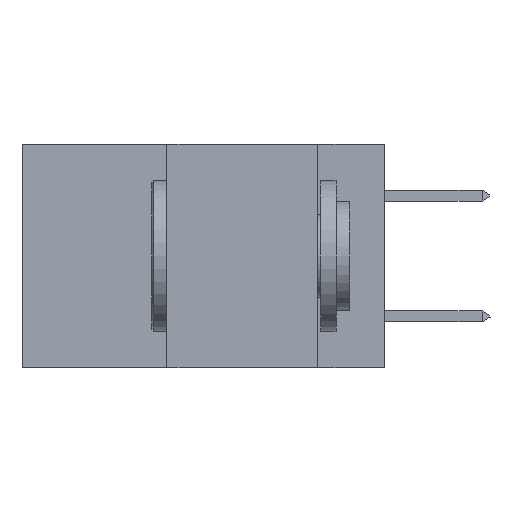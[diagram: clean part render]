
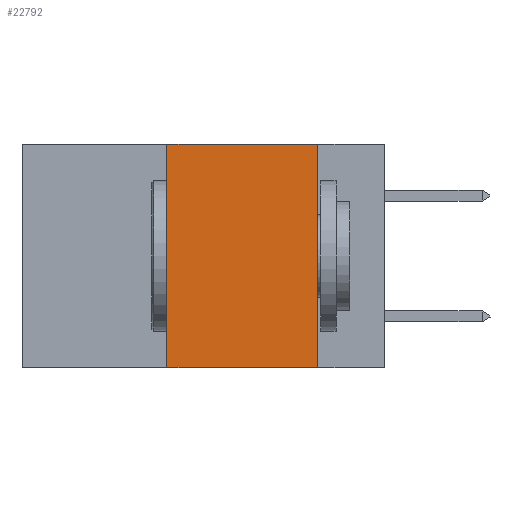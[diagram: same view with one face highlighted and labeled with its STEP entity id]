
A CAD part, left-side view. The second image highlights one B-rep face of the part: STEP entity #22792.
In plain terms, the highlighted planar face has unit normal (-1, 0, 0).
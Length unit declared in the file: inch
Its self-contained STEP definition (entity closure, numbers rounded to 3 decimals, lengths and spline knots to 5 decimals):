
#1737 = AXIS2_PLACEMENT_3D ( 'NONE', #43997, #23491, #2506 ) ;
#1740 = LINE ( 'NONE', #30843, #27474 ) ;
#2506 = DIRECTION ( 'NONE',  ( 0., 0., -1. ) ) ;
#3449 = ORIENTED_EDGE ( 'NONE', *, *, #29821, .T. ) ;
#3748 = VERTEX_POINT ( 'NONE', #8280 ) ;
#5391 = LINE ( 'NONE', #37569, #22908 ) ;
#8248 = DIRECTION ( 'NONE',  ( 0., -1., 0. ) ) ;
#8280 = CARTESIAN_POINT ( 'NONE',  ( 0., 0.36, 0. ) ) ;
#11699 = ORIENTED_EDGE ( 'NONE', *, *, #41206, .F. ) ;
#20995 = DIRECTION ( 'NONE',  ( 0., -1., 0. ) ) ;
#22792 = ADVANCED_FACE ( 'NONE', ( #43495 ), #40586, .F. ) ;
#22908 = VECTOR ( 'NONE', #20995, 39.37008 ) ;
#23491 = DIRECTION ( 'NONE',  ( 1., 0., 0. ) ) ;
#23660 = CARTESIAN_POINT ( 'NONE',  ( 0., 0.36, -0.37 ) ) ;
#25118 = DIRECTION ( 'NONE',  ( 0., 0., 1. ) ) ;
#25657 = CARTESIAN_POINT ( 'NONE',  ( 0., 0.6, 0. ) ) ;
#26062 = VERTEX_POINT ( 'NONE', #23660 ) ;
#27474 = VECTOR ( 'NONE', #34275, 39.37008 ) ;
#27480 = EDGE_CURVE ( 'NONE', #41110, #42711, #1740, .T. ) ;
#27956 = VECTOR ( 'NONE', #8248, 39.37008 ) ;
#29158 = ORIENTED_EDGE ( 'NONE', *, *, #43886, .F. ) ;
#29821 = EDGE_CURVE ( 'NONE', #26062, #42711, #5391, .T. ) ;
#29882 = CARTESIAN_POINT ( 'NONE',  ( 0., 0.11, -0.37 ) ) ;
#30843 = CARTESIAN_POINT ( 'NONE',  ( 0., 0.11, 0. ) ) ;
#34275 = DIRECTION ( 'NONE',  ( 0., 0., -1. ) ) ;
#34899 = CARTESIAN_POINT ( 'NONE',  ( 0., 0.11, 0. ) ) ;
#36461 = LINE ( 'NONE', #42146, #41224 ) ;
#37044 = LINE ( 'NONE', #25657, #27956 ) ;
#37569 = CARTESIAN_POINT ( 'NONE',  ( 0., 0.6, -0.37 ) ) ;
#40586 = PLANE ( 'NONE',  #1737 ) ;
#41015 = EDGE_LOOP ( 'NONE', ( #44065, #29158, #11699, #3449 ) ) ;
#41110 = VERTEX_POINT ( 'NONE', #34899 ) ;
#41206 = EDGE_CURVE ( 'NONE', #26062, #3748, #36461, .T. ) ;
#41224 = VECTOR ( 'NONE', #25118, 39.37008 ) ;
#42146 = CARTESIAN_POINT ( 'NONE',  ( 0., 0.36, 0. ) ) ;
#42711 = VERTEX_POINT ( 'NONE', #29882 ) ;
#43495 = FACE_OUTER_BOUND ( 'NONE', #41015, .T. ) ;
#43886 = EDGE_CURVE ( 'NONE', #3748, #41110, #37044, .T. ) ;
#43997 = CARTESIAN_POINT ( 'NONE',  ( 0., 0.6, 0. ) ) ;
#44065 = ORIENTED_EDGE ( 'NONE', *, *, #27480, .F. ) ;
